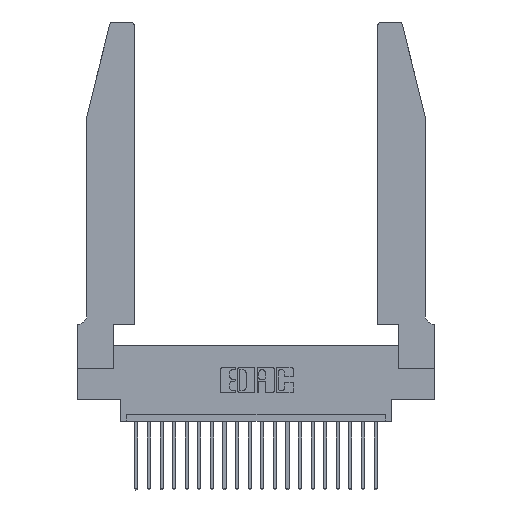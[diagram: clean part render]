
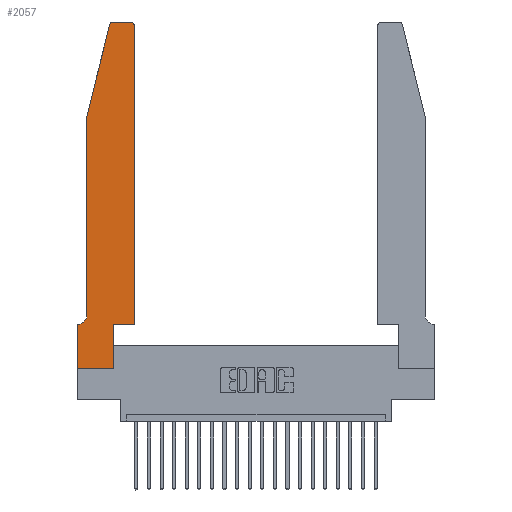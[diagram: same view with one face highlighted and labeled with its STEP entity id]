
A CAD part, top view. The second image highlights one B-rep face of the part: STEP entity #2057.
In plain terms, the highlighted planar face has unit normal (0, 0, 1).
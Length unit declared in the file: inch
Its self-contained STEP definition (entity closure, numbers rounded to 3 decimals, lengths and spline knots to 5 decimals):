
#81 = LINE ( 'NONE', #18096, #6239 ) ;
#289 = CARTESIAN_POINT ( 'NONE',  ( 0.25487, 2.72718, 0.37 ) ) ;
#348 = DIRECTION ( 'NONE',  ( 0., 0., 1. ) ) ;
#864 = EDGE_CURVE ( 'NONE', #1273, #22673, #14351, .T. ) ;
#1273 = VERTEX_POINT ( 'NONE', #15290 ) ;
#1409 = CIRCLE ( 'NONE', #20652, 0.07 ) ;
#1585 = CIRCLE ( 'NONE', #6135, 0.03 ) ;
#2057 = ADVANCED_FACE ( 'NONE', ( #19837 ), #14576, .T. ) ;
#2278 = DIRECTION ( 'NONE',  ( 1., 0., 0. ) ) ;
#2456 = CARTESIAN_POINT ( 'NONE',  ( 0.4505, 0.35, 0.37 ) ) ;
#2469 = CARTESIAN_POINT ( 'NONE',  ( 0.0055, 0.35, 0.37 ) ) ;
#3328 = CARTESIAN_POINT ( 'NONE',  ( 0.4505, 0.35, 0.37 ) ) ;
#3433 = VECTOR ( 'NONE', #12320, 39.37008 ) ;
#3468 = AXIS2_PLACEMENT_3D ( 'NONE', #7762, #14678, #20251 ) ;
#3753 = EDGE_CURVE ( 'NONE', #16531, #19295, #1585, .T. ) ;
#4293 = EDGE_CURVE ( 'NONE', #17931, #17339, #22060, .T. ) ;
#4387 = CARTESIAN_POINT ( 'NONE',  ( 0.2865, 0.35, 0.37 ) ) ;
#4477 = EDGE_CURVE ( 'NONE', #4826, #5147, #12926, .T. ) ;
#4699 = ORIENTED_EDGE ( 'NONE', *, *, #12448, .T. ) ;
#4826 = VERTEX_POINT ( 'NONE', #11892 ) ;
#5147 = VERTEX_POINT ( 'NONE', #289 ) ;
#5471 = ORIENTED_EDGE ( 'NONE', *, *, #4477, .T. ) ;
#5945 = DIRECTION ( 'NONE',  ( -1., 0., 0. ) ) ;
#6010 = DIRECTION ( 'NONE',  ( 0., 1., 0. ) ) ;
#6135 = AXIS2_PLACEMENT_3D ( 'NONE', #16281, #19783, #9222 ) ;
#6192 = VECTOR ( 'NONE', #6658, 39.37008 ) ;
#6239 = VECTOR ( 'NONE', #21741, 39.37008 ) ;
#6353 = VECTOR ( 'NONE', #22385, 39.37008 ) ;
#6658 = DIRECTION ( 'NONE',  ( -0.239, -0.971, 0. ) ) ;
#6804 = CARTESIAN_POINT ( 'NONE',  ( 0.0755, 0.35, 0.37 ) ) ;
#6860 = ORIENTED_EDGE ( 'NONE', *, *, #21958, .T. ) ;
#7003 = CARTESIAN_POINT ( 'NONE',  ( 0.2605, 2.75, 0.37 ) ) ;
#7239 = EDGE_CURVE ( 'NONE', #22673, #17931, #1409, .T. ) ;
#7762 = CARTESIAN_POINT ( 'NONE',  ( 0.284, 2.72, 0.37 ) ) ;
#7882 = LINE ( 'NONE', #11913, #15566 ) ;
#8249 = VECTOR ( 'NONE', #5945, 39.37008 ) ;
#8254 = ORIENTED_EDGE ( 'NONE', *, *, #3753, .T. ) ;
#9206 = AXIS2_PLACEMENT_3D ( 'NONE', #21563, #348, #2278 ) ;
#9222 = DIRECTION ( 'NONE',  ( 1., 0., 0. ) ) ;
#9474 = VERTEX_POINT ( 'NONE', #3328 ) ;
#10384 = ORIENTED_EDGE ( 'NONE', *, *, #4293, .T. ) ;
#10783 = ORIENTED_EDGE ( 'NONE', *, *, #7239, .T. ) ;
#10913 = ORIENTED_EDGE ( 'NONE', *, *, #22242, .T. ) ;
#11145 = VECTOR ( 'NONE', #19463, 39.37008 ) ;
#11198 = CARTESIAN_POINT ( 'NONE',  ( 0., 0., 0.37 ) ) ;
#11509 = LINE ( 'NONE', #2456, #21719 ) ;
#11892 = CARTESIAN_POINT ( 'NONE',  ( 0.284, 2.75, 0.37 ) ) ;
#11913 = CARTESIAN_POINT ( 'NONE',  ( 0.4505, 0.35, 0.37 ) ) ;
#12006 = LINE ( 'NONE', #7003, #18596 ) ;
#12320 = DIRECTION ( 'NONE',  ( 1., 0., 0. ) ) ;
#12339 = DIRECTION ( 'NONE',  ( -1., 0., 0. ) ) ;
#12448 = EDGE_CURVE ( 'NONE', #19295, #4826, #12006, .T. ) ;
#12926 = CIRCLE ( 'NONE', #3468, 0.03 ) ;
#13029 = CARTESIAN_POINT ( 'NONE',  ( 0., 0.35, 0.37 ) ) ;
#13645 = CARTESIAN_POINT ( 'NONE',  ( 0.0755, 2., 0.37 ) ) ;
#13776 = EDGE_CURVE ( 'NONE', #17441, #17372, #81, .T. ) ;
#13907 = CARTESIAN_POINT ( 'NONE',  ( 0.4505, 2.72, 0.37 ) ) ;
#14351 = LINE ( 'NONE', #13645, #6353 ) ;
#14576 = PLANE ( 'NONE',  #9206 ) ;
#14678 = DIRECTION ( 'NONE',  ( 0., 0., 1. ) ) ;
#14803 = EDGE_CURVE ( 'NONE', #17339, #17421, #19978, .T. ) ;
#14911 = CARTESIAN_POINT ( 'NONE',  ( 0.0055, 0.42, 0.37 ) ) ;
#15166 = CARTESIAN_POINT ( 'NONE',  ( 0.2865, 0., 0.37 ) ) ;
#15290 = CARTESIAN_POINT ( 'NONE',  ( 0.0755, 2., 0.37 ) ) ;
#15566 = VECTOR ( 'NONE', #17205, 39.37008 ) ;
#16281 = CARTESIAN_POINT ( 'NONE',  ( 0.4205, 2.72, 0.37 ) ) ;
#16445 = CARTESIAN_POINT ( 'NONE',  ( 0.4205, 2.75, 0.37 ) ) ;
#16531 = VERTEX_POINT ( 'NONE', #13907 ) ;
#16835 = DIRECTION ( 'NONE',  ( 0., 0., -1. ) ) ;
#16966 = CARTESIAN_POINT ( 'NONE',  ( 0.0755, 0.42, 0.37 ) ) ;
#17097 = EDGE_CURVE ( 'NONE', #5147, #1273, #22466, .T. ) ;
#17205 = DIRECTION ( 'NONE',  ( 1., 0., 0. ) ) ;
#17339 = VERTEX_POINT ( 'NONE', #13029 ) ;
#17372 = VERTEX_POINT ( 'NONE', #4387 ) ;
#17421 = VERTEX_POINT ( 'NONE', #11198 ) ;
#17441 = VERTEX_POINT ( 'NONE', #15166 ) ;
#17609 = CARTESIAN_POINT ( 'NONE',  ( 0., 0., 0.37 ) ) ;
#17931 = VERTEX_POINT ( 'NONE', #2469 ) ;
#18070 = ORIENTED_EDGE ( 'NONE', *, *, #17097, .T. ) ;
#18096 = CARTESIAN_POINT ( 'NONE',  ( 0.2865, 0.35, 0.37 ) ) ;
#18552 = DIRECTION ( 'NONE',  ( -1., 0., 0. ) ) ;
#18596 = VECTOR ( 'NONE', #12339, 39.37008 ) ;
#19162 = CARTESIAN_POINT ( 'NONE',  ( 0., 0., 0.37 ) ) ;
#19295 = VERTEX_POINT ( 'NONE', #16445 ) ;
#19463 = DIRECTION ( 'NONE',  ( 0., -1., 0. ) ) ;
#19783 = DIRECTION ( 'NONE',  ( 0., 0., 1. ) ) ;
#19837 = FACE_OUTER_BOUND ( 'NONE', #20825, .T. ) ;
#19978 = LINE ( 'NONE', #17609, #11145 ) ;
#20251 = DIRECTION ( 'NONE',  ( 1., 0., 0. ) ) ;
#20652 = AXIS2_PLACEMENT_3D ( 'NONE', #14911, #16835, #18552 ) ;
#20825 = EDGE_LOOP ( 'NONE', ( #4699, #5471, #18070, #21658, #10783, #10384, #22079, #10913, #21881, #22076, #6860, #8254 ) ) ;
#21563 = CARTESIAN_POINT ( 'NONE',  ( 0., 0.35, 0.37 ) ) ;
#21658 = ORIENTED_EDGE ( 'NONE', *, *, #864, .T. ) ;
#21719 = VECTOR ( 'NONE', #6010, 39.37008 ) ;
#21741 = DIRECTION ( 'NONE',  ( 0., 1., 0. ) ) ;
#21881 = ORIENTED_EDGE ( 'NONE', *, *, #13776, .T. ) ;
#21958 = EDGE_CURVE ( 'NONE', #9474, #16531, #11509, .T. ) ;
#22060 = LINE ( 'NONE', #6804, #8249 ) ;
#22076 = ORIENTED_EDGE ( 'NONE', *, *, #22681, .T. ) ;
#22079 = ORIENTED_EDGE ( 'NONE', *, *, #14803, .T. ) ;
#22242 = EDGE_CURVE ( 'NONE', #17421, #17441, #22249, .T. ) ;
#22249 = LINE ( 'NONE', #19162, #3433 ) ;
#22385 = DIRECTION ( 'NONE',  ( 0., -1., 0. ) ) ;
#22466 = LINE ( 'NONE', #22490, #6192 ) ;
#22490 = CARTESIAN_POINT ( 'NONE',  ( 0.0755, 2., 0.37 ) ) ;
#22673 = VERTEX_POINT ( 'NONE', #16966 ) ;
#22681 = EDGE_CURVE ( 'NONE', #17372, #9474, #7882, .T. ) ;
